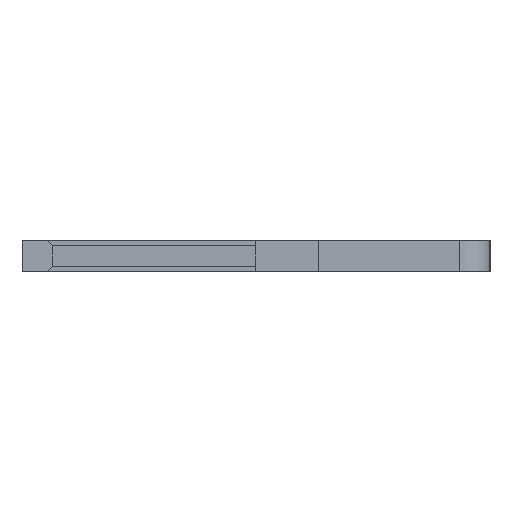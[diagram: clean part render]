
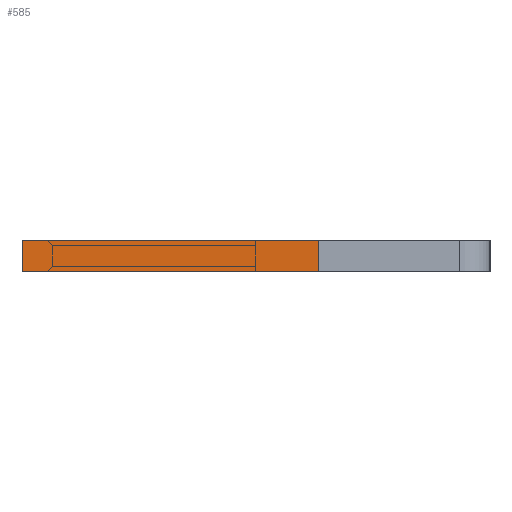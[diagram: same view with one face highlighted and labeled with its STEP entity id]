
A CAD part, left-side view. The second image highlights one B-rep face of the part: STEP entity #585.
In plain terms, the highlighted face is planar.
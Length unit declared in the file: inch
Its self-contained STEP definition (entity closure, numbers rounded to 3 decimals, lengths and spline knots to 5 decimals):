
#9 = VECTOR ( 'NONE', #3203, 39.37008 ) ;
#78 = CARTESIAN_POINT ( 'NONE',  ( -0.01, 0.15, -0.04 ) ) ;
#102 = PLANE ( 'NONE',  #1150 ) ;
#177 = ORIENTED_EDGE ( 'NONE', *, *, #1701, .F. ) ;
#331 = DIRECTION ( 'NONE',  ( 1., 0., 0. ) ) ;
#345 = VECTOR ( 'NONE', #2180, 39.37008 ) ;
#400 = VERTEX_POINT ( 'NONE', #2589 ) ;
#480 = CARTESIAN_POINT ( 'NONE',  ( -0.01, -0.04, -0.04 ) ) ;
#545 = CARTESIAN_POINT ( 'NONE',  ( 0.01, 0.15, -0.04 ) ) ;
#585 = ADVANCED_FACE ( 'NONE', ( #1010 ), #102, .F. ) ;
#619 = LINE ( 'NONE', #545, #1948 ) ;
#635 = CARTESIAN_POINT ( 'NONE',  ( 0.01, 0.15, -0.04 ) ) ;
#661 = DIRECTION ( 'NONE',  ( 0., 0., 1. ) ) ;
#668 = VERTEX_POINT ( 'NONE', #2065 ) ;
#731 = CARTESIAN_POINT ( 'NONE',  ( 0.01, -0.04, -0.04 ) ) ;
#746 = EDGE_CURVE ( 'NONE', #1102, #400, #1559, .T. ) ;
#930 = ORIENTED_EDGE ( 'NONE', *, *, #2504, .F. ) ;
#1010 = FACE_OUTER_BOUND ( 'NONE', #1511, .T. ) ;
#1091 = LINE ( 'NONE', #731, #345 ) ;
#1102 = VERTEX_POINT ( 'NONE', #480 ) ;
#1145 = ORIENTED_EDGE ( 'NONE', *, *, #746, .T. ) ;
#1150 = AXIS2_PLACEMENT_3D ( 'NONE', #635, #661, #331 ) ;
#1511 = EDGE_LOOP ( 'NONE', ( #1145, #177, #930, #2355 ) ) ;
#1559 = LINE ( 'NONE', #78, #9 ) ;
#1646 = DIRECTION ( 'NONE',  ( -1., 0., 0. ) ) ;
#1701 = EDGE_CURVE ( 'NONE', #668, #400, #619, .T. ) ;
#1948 = VECTOR ( 'NONE', #1646, 39.37008 ) ;
#1950 = DIRECTION ( 'NONE',  ( 0., 1., 0. ) ) ;
#1993 = LINE ( 'NONE', #2773, #3395 ) ;
#2065 = CARTESIAN_POINT ( 'NONE',  ( 0.01, 0.15, -0.04 ) ) ;
#2180 = DIRECTION ( 'NONE',  ( -1., 0., 0. ) ) ;
#2200 = EDGE_CURVE ( 'NONE', #2621, #1102, #1091, .T. ) ;
#2355 = ORIENTED_EDGE ( 'NONE', *, *, #2200, .T. ) ;
#2504 = EDGE_CURVE ( 'NONE', #2621, #668, #1993, .T. ) ;
#2589 = CARTESIAN_POINT ( 'NONE',  ( -0.01, 0.15, -0.04 ) ) ;
#2621 = VERTEX_POINT ( 'NONE', #3084 ) ;
#2773 = CARTESIAN_POINT ( 'NONE',  ( 0.01, 0.15, -0.04 ) ) ;
#3084 = CARTESIAN_POINT ( 'NONE',  ( 0.01, -0.04, -0.04 ) ) ;
#3203 = DIRECTION ( 'NONE',  ( 0., 1., 0. ) ) ;
#3395 = VECTOR ( 'NONE', #1950, 39.37008 ) ;
